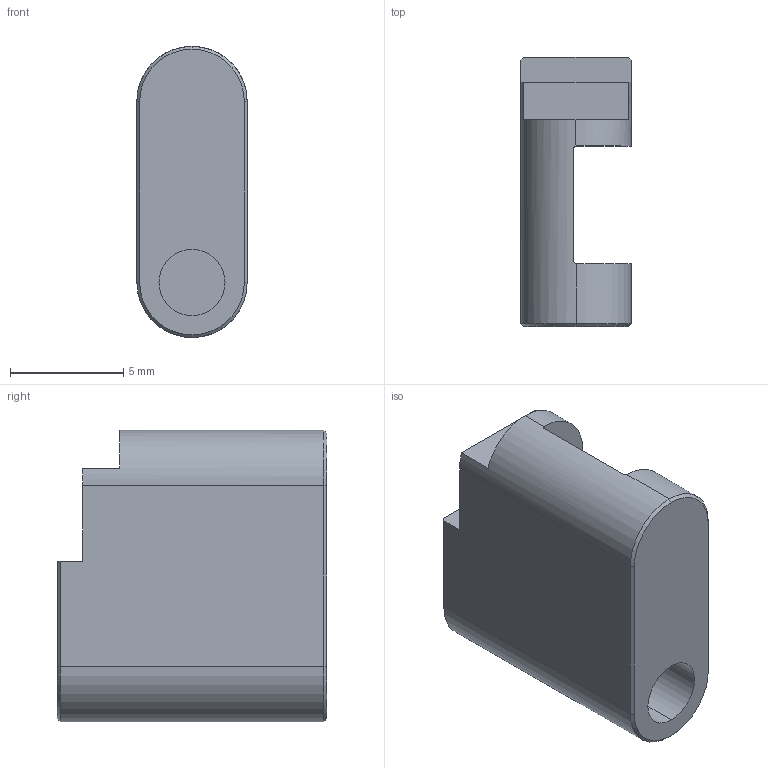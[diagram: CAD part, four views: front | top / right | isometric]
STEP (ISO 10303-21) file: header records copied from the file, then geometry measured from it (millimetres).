
FILE_DESCRIPTION (( 'STEP AP214' ), '1' );
FILE_NAME ('STRIKER SAFETY.STEP', '2013-06-19T13:56:51', ( 'Asher' ), ( '' ), 'SwSTEP 2.0', 'SolidWorks 2013', '' );
FILE_SCHEMA (( 'AUTOMOTIVE_DESIGN' ));
Length unit declared in the file: millimetre
Products named in the file (1): STRIKER SAFETY
Bounding box: 4.88 x 11.91 x 12.88 mm (x, y, z)
Volume: 474.9 mm3; surface area: 538.5 mm2
Topology: 1 solids, 1 shells, 30 faces, 74 edges, 47 vertices
Faces by surface type: plane 17, cylinder 8, cone 5
Entity records: 972 total; most frequent: CARTESIAN_POINT 218, DIRECTION 152, ORIENTED_EDGE 148, EDGE_CURVE 74, AXIS2_PLACEMENT_3D 53, VERTEX_POINT 47, VECTOR 46, LINE 46
